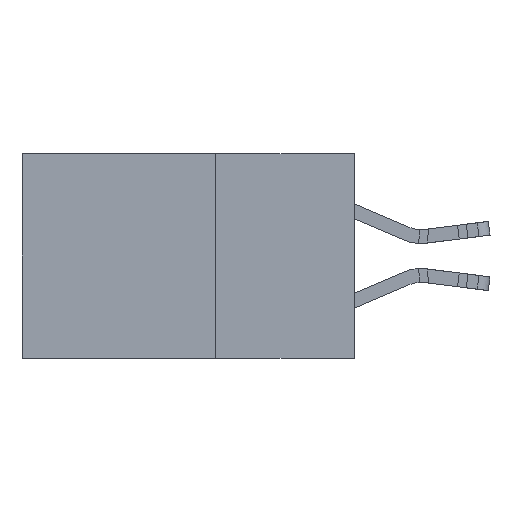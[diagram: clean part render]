
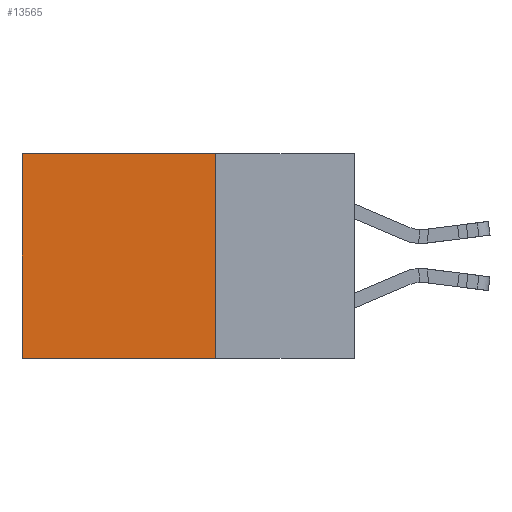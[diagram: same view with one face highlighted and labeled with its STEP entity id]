
A CAD part, left-side view. The second image highlights one B-rep face of the part: STEP entity #13565.
In plain terms, the highlighted planar face has unit normal (-1, 0, 0).
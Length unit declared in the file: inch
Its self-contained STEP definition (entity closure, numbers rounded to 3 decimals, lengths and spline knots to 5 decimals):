
#1273 = LINE ( 'NONE', #16504, #3638 ) ;
#1314 = DIRECTION ( 'NONE',  ( 0., 1., 0. ) ) ;
#2971 = EDGE_CURVE ( 'NONE', #7120, #17430, #12020, .T. ) ;
#3638 = VECTOR ( 'NONE', #1314, 39.37008 ) ;
#5241 = VECTOR ( 'NONE', #8788, 39.37008 ) ;
#5662 = LINE ( 'NONE', #15912, #30686 ) ;
#6054 = VERTEX_POINT ( 'NONE', #25467 ) ;
#6511 = DIRECTION ( 'NONE',  ( 0., 0., -1. ) ) ;
#6894 = DIRECTION ( 'NONE',  ( 0., 0., -1. ) ) ;
#7120 = VERTEX_POINT ( 'NONE', #15552 ) ;
#8633 = CARTESIAN_POINT ( 'NONE',  ( 0.298, 0.25, 0. ) ) ;
#8729 = EDGE_LOOP ( 'NONE', ( #21252, #16039, #8986, #17089 ) ) ;
#8788 = DIRECTION ( 'NONE',  ( 0., 1., 0. ) ) ;
#8986 = ORIENTED_EDGE ( 'NONE', *, *, #29000, .F. ) ;
#9023 = DIRECTION ( 'NONE',  ( 1., 0., 0. ) ) ;
#11041 = AXIS2_PLACEMENT_3D ( 'NONE', #27199, #9023, #6894 ) ;
#11727 = FACE_OUTER_BOUND ( 'NONE', #8729, .T. ) ;
#12020 = LINE ( 'NONE', #24101, #5241 ) ;
#13565 = ADVANCED_FACE ( 'NONE', ( #11727 ), #16771, .F. ) ;
#15544 = LINE ( 'NONE', #8633, #20719 ) ;
#15552 = CARTESIAN_POINT ( 'NONE',  ( 0.298, 0.25, -0.37 ) ) ;
#15912 = CARTESIAN_POINT ( 'NONE',  ( 0.298, 0.6, 0. ) ) ;
#16017 = DIRECTION ( 'NONE',  ( 0., 0., -1. ) ) ;
#16039 = ORIENTED_EDGE ( 'NONE', *, *, #2971, .F. ) ;
#16504 = CARTESIAN_POINT ( 'NONE',  ( 0.298, 0.25, 0. ) ) ;
#16526 = CARTESIAN_POINT ( 'NONE',  ( 0.298, 0.6, -0.37 ) ) ;
#16771 = PLANE ( 'NONE',  #11041 ) ;
#17089 = ORIENTED_EDGE ( 'NONE', *, *, #29013, .T. ) ;
#17227 = CARTESIAN_POINT ( 'NONE',  ( 0.298, 0.6, 0. ) ) ;
#17430 = VERTEX_POINT ( 'NONE', #16526 ) ;
#18997 = VERTEX_POINT ( 'NONE', #17227 ) ;
#20719 = VECTOR ( 'NONE', #6511, 39.37008 ) ;
#21252 = ORIENTED_EDGE ( 'NONE', *, *, #23920, .T. ) ;
#23920 = EDGE_CURVE ( 'NONE', #18997, #17430, #5662, .T. ) ;
#24101 = CARTESIAN_POINT ( 'NONE',  ( 0.298, 0.25, -0.37 ) ) ;
#25467 = CARTESIAN_POINT ( 'NONE',  ( 0.298, 0.25, 0. ) ) ;
#27199 = CARTESIAN_POINT ( 'NONE',  ( 0.298, 0.25, 0. ) ) ;
#29000 = EDGE_CURVE ( 'NONE', #6054, #7120, #15544, .T. ) ;
#29013 = EDGE_CURVE ( 'NONE', #6054, #18997, #1273, .T. ) ;
#30686 = VECTOR ( 'NONE', #16017, 39.37008 ) ;
